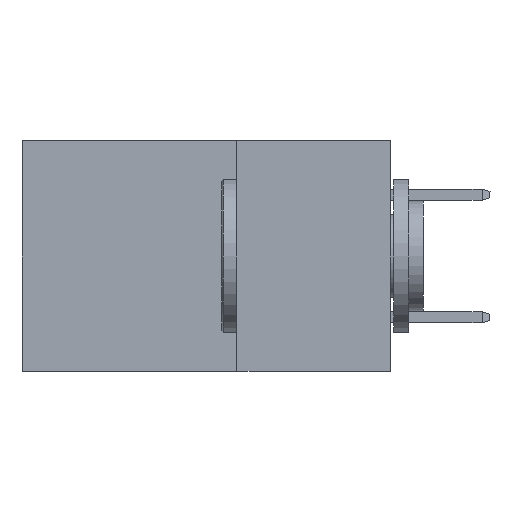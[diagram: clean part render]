
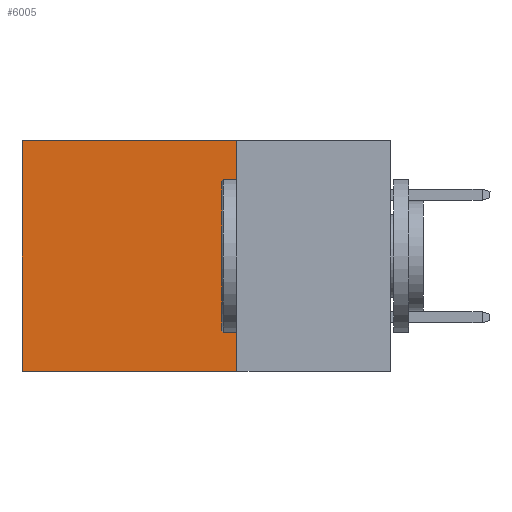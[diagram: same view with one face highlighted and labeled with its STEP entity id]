
A CAD part, left-side view. The second image highlights one B-rep face of the part: STEP entity #6005.
In plain terms, the highlighted planar face has unit normal (-1, 0, 0).
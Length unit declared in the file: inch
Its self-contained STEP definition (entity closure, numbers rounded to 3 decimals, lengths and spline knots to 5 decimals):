
#547 = ORIENTED_EDGE ( 'NONE', *, *, #2078, .F. ) ;
#682 = PLANE ( 'NONE',  #6915 ) ;
#724 = VECTOR ( 'NONE', #4291, 39.37008 ) ;
#1099 = ORIENTED_EDGE ( 'NONE', *, *, #8757, .F. ) ;
#1538 = DIRECTION ( 'NONE',  ( 0., 1., 0. ) ) ;
#1745 = LINE ( 'NONE', #5579, #5301 ) ;
#1758 = CARTESIAN_POINT ( 'NONE',  ( 0.2875, 0.25, -0.375 ) ) ;
#1792 = CARTESIAN_POINT ( 'NONE',  ( 0.2875, 0.25, -0.375 ) ) ;
#2078 = EDGE_CURVE ( 'NONE', #4402, #2104, #5519, .T. ) ;
#2104 = VERTEX_POINT ( 'NONE', #1758 ) ;
#2202 = VERTEX_POINT ( 'NONE', #3313 ) ;
#2250 = CARTESIAN_POINT ( 'NONE',  ( 0.2875, 0.25, 0. ) ) ;
#2501 = DIRECTION ( 'NONE',  ( 0., 0., -1. ) ) ;
#2983 = DIRECTION ( 'NONE',  ( 1., 0., 0. ) ) ;
#3313 = CARTESIAN_POINT ( 'NONE',  ( 0.2875, 0.6, -0.375 ) ) ;
#3368 = VECTOR ( 'NONE', #1538, 39.37008 ) ;
#4113 = CARTESIAN_POINT ( 'NONE',  ( 0.2875, 0.6, 0. ) ) ;
#4291 = DIRECTION ( 'NONE',  ( 0., 0., -1. ) ) ;
#4402 = VERTEX_POINT ( 'NONE', #2250 ) ;
#4583 = ORIENTED_EDGE ( 'NONE', *, *, #5383, .T. ) ;
#4905 = EDGE_CURVE ( 'NONE', #4402, #8650, #1745, .T. ) ;
#5301 = VECTOR ( 'NONE', #7730, 39.37008 ) ;
#5383 = EDGE_CURVE ( 'NONE', #8650, #2202, #6435, .T. ) ;
#5519 = LINE ( 'NONE', #1792, #8003 ) ;
#5579 = CARTESIAN_POINT ( 'NONE',  ( 0.2875, 0.25, 0. ) ) ;
#5679 = CARTESIAN_POINT ( 'NONE',  ( 0.2875, 0.25, -0.375 ) ) ;
#5812 = CARTESIAN_POINT ( 'NONE',  ( 0.2875, 0.6, -0.375 ) ) ;
#6005 = ADVANCED_FACE ( 'NONE', ( #6308 ), #682, .F. ) ;
#6308 = FACE_OUTER_BOUND ( 'NONE', #7736, .T. ) ;
#6435 = LINE ( 'NONE', #5812, #724 ) ;
#6437 = CARTESIAN_POINT ( 'NONE',  ( 0.2875, 0.25, -0.375 ) ) ;
#6915 = AXIS2_PLACEMENT_3D ( 'NONE', #5679, #2983, #8006 ) ;
#7730 = DIRECTION ( 'NONE',  ( 0., 1., 0. ) ) ;
#7736 = EDGE_LOOP ( 'NONE', ( #4583, #1099, #547, #8870 ) ) ;
#8003 = VECTOR ( 'NONE', #2501, 39.37008 ) ;
#8006 = DIRECTION ( 'NONE',  ( 0., 0., -1. ) ) ;
#8650 = VERTEX_POINT ( 'NONE', #4113 ) ;
#8757 = EDGE_CURVE ( 'NONE', #2104, #2202, #8846, .T. ) ;
#8846 = LINE ( 'NONE', #6437, #3368 ) ;
#8870 = ORIENTED_EDGE ( 'NONE', *, *, #4905, .T. ) ;
